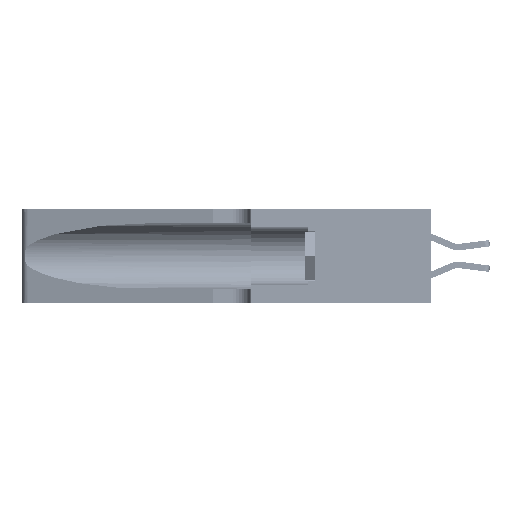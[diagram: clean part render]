
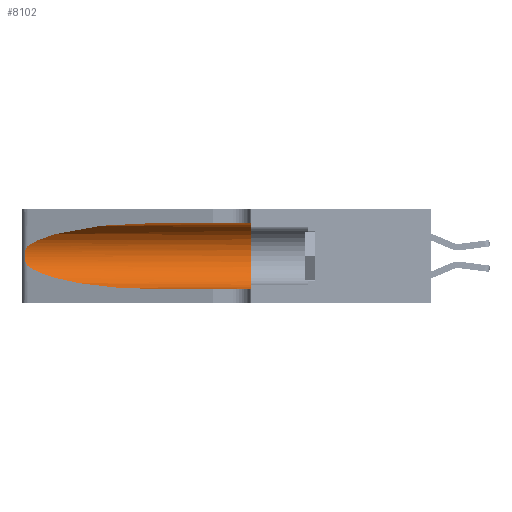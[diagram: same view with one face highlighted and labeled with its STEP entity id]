
A CAD part, left-side view. The second image highlights one B-rep face of the part: STEP entity #8102.
In plain terms, the highlighted cylindrical face has radius 3.308 mm (diameter 6.617 mm), a partial arc.
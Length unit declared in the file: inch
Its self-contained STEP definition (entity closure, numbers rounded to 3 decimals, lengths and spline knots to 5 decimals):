
#1662 = CARTESIAN_POINT ( 'NONE',  ( 0.1305, 0.72297, 0.05475 ) ) ;
#2196 = CARTESIAN_POINT ( 'NONE',  ( 0.26075, 1.23896, 0.19203 ) ) ;
#2498 = FACE_OUTER_BOUND ( 'NONE', #17645, .T. ) ;
#3041 = VERTEX_POINT ( 'NONE', #19536 ) ;
#4347 = CARTESIAN_POINT ( 'NONE',  ( 0.1305, 1.61858, 0.185 ) ) ;
#5514 = CARTESIAN_POINT ( 'NONE',  ( 0.26017, 1.23833, 0.17102 ) ) ;
#6642 = EDGE_CURVE ( 'NONE', #3041, #35094, #15085, .T. ) ;
#6744 = EDGE_CURVE ( 'NONE', #3041, #33937, #36654, .T. ) ;
#6959 = CARTESIAN_POINT ( 'NONE',  ( 0.1305, 1.61858, 0.05475 ) ) ;
#8098 = CYLINDRICAL_SURFACE ( 'NONE', #32248, 0.13025 ) ;
#8102 = ADVANCED_FACE ( 'NONE', ( #2498 ), #8098, .F. ) ;
#8758 = CARTESIAN_POINT ( 'NONE',  ( 0.25789, 1.23486, 0.15765 ) ) ;
#8915 =( BOUNDED_CURVE ( )  B_SPLINE_CURVE ( 3, ( #17740, #14534, #20944, #1662 ),
 .UNSPECIFIED., .F., .T. ) 
 B_SPLINE_CURVE_WITH_KNOTS ( ( 4, 4 ),
 ( 3.44316, 4.71239 ),
 .UNSPECIFIED. ) 
 CURVE ( )  GEOMETRIC_REPRESENTATION_ITEM ( )  RATIONAL_B_SPLINE_CURVE ( ( 1., 0.87, 0.87, 1. ) ) 
 REPRESENTATION_ITEM ( '' )  );
#11107 = DIRECTION ( 'NONE',  ( 0., 1., 0. ) ) ;
#11997 = CARTESIAN_POINT ( 'NONE',  ( 0.25555, 1.22993, 0.14849 ) ) ;
#12803 = CARTESIAN_POINT ( 'NONE',  ( 0.1305, 0.35, 0.05475 ) ) ;
#13767 = CARTESIAN_POINT ( 'NONE',  ( 0.1305, 1.61858, 0.31525 ) ) ;
#14255 = VECTOR ( 'NONE', #22687, 39.37008 ) ;
#14534 = CARTESIAN_POINT ( 'NONE',  ( 0.2373, 1.15595, 0.08982 ) ) ;
#15070 = CARTESIAN_POINT ( 'NONE',  ( 0.25487, 1.22718, 0.22369 ) ) ;
#15085 =( BOUNDED_CURVE ( )  B_SPLINE_CURVE ( 3, ( #34920, #15880, #38107, #19071 ),
 .UNSPECIFIED., .F., .T. ) 
 B_SPLINE_CURVE_WITH_KNOTS ( ( 4, 4 ),
 ( 1.5708, 2.84003 ),
 .UNSPECIFIED. ) 
 CURVE ( )  GEOMETRIC_REPRESENTATION_ITEM ( )  RATIONAL_B_SPLINE_CURVE ( ( 1., 0.87, 0.87, 1. ) ) 
 REPRESENTATION_ITEM ( '' )  );
#15880 = CARTESIAN_POINT ( 'NONE',  ( 0.18966, 0.96281, 0.31525 ) ) ;
#16384 = B_SPLINE_CURVE_WITH_KNOTS ( 'NONE', 3,
 ( #15070, #34115, #37325, #18284, #40509, #21491, #2196, #24693, #5514, #27891, #8758, #31062, #11997, #34263 ),
 .UNSPECIFIED., .F., .F.,
 ( 4, 2, 2, 2, 2, 2, 4 ),
 ( 0., 0.00027, 0.00053, 0.00107, 0.0016, 0.00187, 0.00214 ),
 .UNSPECIFIED. ) ;
#16682 = ORIENTED_EDGE ( 'NONE', *, *, #6642, .T. ) ;
#17139 = EDGE_CURVE ( 'NONE', #33937, #34511, #22231, .T. ) ;
#17186 = ORIENTED_EDGE ( 'NONE', *, *, #6744, .F. ) ;
#17645 = EDGE_LOOP ( 'NONE', ( #16682, #28138, #36563, #22666, #39542, #17186 ) ) ;
#17740 = CARTESIAN_POINT ( 'NONE',  ( 0.25487, 1.22718, 0.14631 ) ) ;
#18042 = AXIS2_PLACEMENT_3D ( 'NONE', #30196, #11107, #33381 ) ;
#18053 = CARTESIAN_POINT ( 'NONE',  ( 0.25487, 1.22718, 0.14631 ) ) ;
#18284 = CARTESIAN_POINT ( 'NONE',  ( 0.25787, 1.23484, 0.2124 ) ) ;
#19071 = CARTESIAN_POINT ( 'NONE',  ( 0.25487, 1.22718, 0.22369 ) ) ;
#19536 = CARTESIAN_POINT ( 'NONE',  ( 0.1305, 0.72297, 0.31525 ) ) ;
#20944 = CARTESIAN_POINT ( 'NONE',  ( 0.18966, 0.96281, 0.05475 ) ) ;
#21491 = CARTESIAN_POINT ( 'NONE',  ( 0.26018, 1.23835, 0.19895 ) ) ;
#22231 = CIRCLE ( 'NONE', #18042, 0.13025 ) ;
#22666 = ORIENTED_EDGE ( 'NONE', *, *, #40673, .T. ) ;
#22687 = DIRECTION ( 'NONE',  ( 0., -1., 0. ) ) ;
#22836 = VERTEX_POINT ( 'NONE', #25476 ) ;
#24534 = VERTEX_POINT ( 'NONE', #18053 ) ;
#24693 = CARTESIAN_POINT ( 'NONE',  ( 0.26075, 1.23896, 0.178 ) ) ;
#25269 = EDGE_CURVE ( 'NONE', #35094, #24534, #16384, .T. ) ;
#25476 = CARTESIAN_POINT ( 'NONE',  ( 0.1305, 0.72297, 0.05475 ) ) ;
#26613 = VECTOR ( 'NONE', #32467, 39.37008 ) ;
#27322 = EDGE_CURVE ( 'NONE', #24534, #22836, #8915, .T. ) ;
#27891 = CARTESIAN_POINT ( 'NONE',  ( 0.25856, 1.23593, 0.16098 ) ) ;
#28138 = ORIENTED_EDGE ( 'NONE', *, *, #25269, .T. ) ;
#30196 = CARTESIAN_POINT ( 'NONE',  ( 0.1305, 0.35, 0.185 ) ) ;
#31062 = CARTESIAN_POINT ( 'NONE',  ( 0.25639, 1.23186, 0.15144 ) ) ;
#31260 = CARTESIAN_POINT ( 'NONE',  ( 0.25487, 1.22718, 0.22369 ) ) ;
#32248 = AXIS2_PLACEMENT_3D ( 'NONE', #4347, #33117, #39509 ) ;
#32467 = DIRECTION ( 'NONE',  ( 0., -1., 0. ) ) ;
#33117 = DIRECTION ( 'NONE',  ( 0., -1., 0. ) ) ;
#33381 = DIRECTION ( 'NONE',  ( 0., 0., 1. ) ) ;
#33937 = VERTEX_POINT ( 'NONE', #34956 ) ;
#34115 = CARTESIAN_POINT ( 'NONE',  ( 0.25555, 1.22994, 0.2215 ) ) ;
#34263 = CARTESIAN_POINT ( 'NONE',  ( 0.25487, 1.22718, 0.14631 ) ) ;
#34511 = VERTEX_POINT ( 'NONE', #12803 ) ;
#34920 = CARTESIAN_POINT ( 'NONE',  ( 0.1305, 0.72297, 0.31525 ) ) ;
#34956 = CARTESIAN_POINT ( 'NONE',  ( 0.1305, 0.35, 0.31525 ) ) ;
#35073 = LINE ( 'NONE', #6959, #26613 ) ;
#35094 = VERTEX_POINT ( 'NONE', #31260 ) ;
#36563 = ORIENTED_EDGE ( 'NONE', *, *, #27322, .T. ) ;
#36654 = LINE ( 'NONE', #13767, #14255 ) ;
#37325 = CARTESIAN_POINT ( 'NONE',  ( 0.25639, 1.23184, 0.21858 ) ) ;
#38107 = CARTESIAN_POINT ( 'NONE',  ( 0.2373, 1.15595, 0.28018 ) ) ;
#39509 = DIRECTION ( 'NONE',  ( 0., 0., -1. ) ) ;
#39542 = ORIENTED_EDGE ( 'NONE', *, *, #17139, .F. ) ;
#40509 = CARTESIAN_POINT ( 'NONE',  ( 0.25854, 1.2359, 0.20912 ) ) ;
#40673 = EDGE_CURVE ( 'NONE', #22836, #34511, #35073, .T. ) ;
